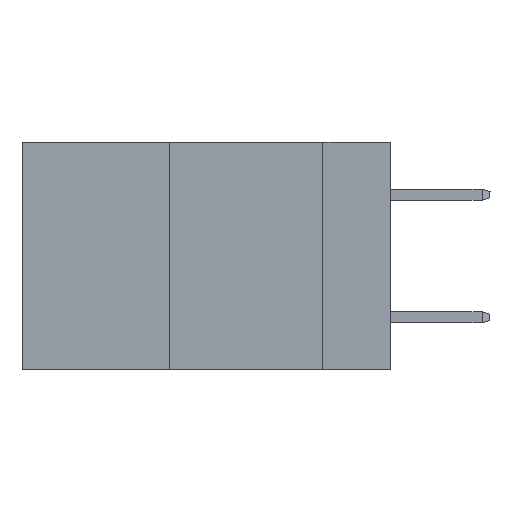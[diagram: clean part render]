
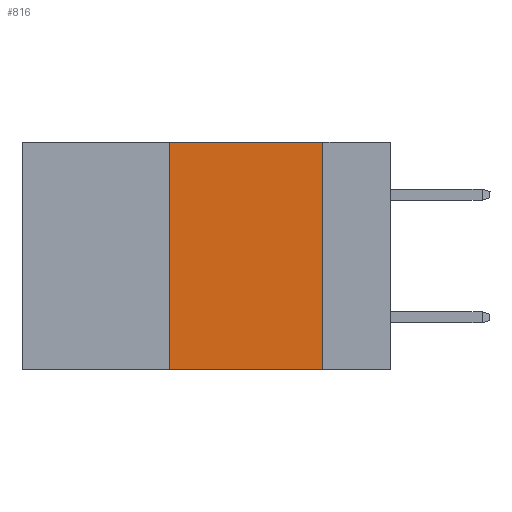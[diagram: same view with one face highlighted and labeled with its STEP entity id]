
A CAD part, left-side view. The second image highlights one B-rep face of the part: STEP entity #816.
In plain terms, the highlighted planar face has unit normal (-1, 0, 0).
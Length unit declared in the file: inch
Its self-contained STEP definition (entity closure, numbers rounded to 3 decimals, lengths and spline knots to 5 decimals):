
#351 = PLANE ( 'NONE',  #15941 ) ;
#454 = EDGE_CURVE ( 'NONE', #11576, #11457, #7574, .T. ) ;
#580 = LINE ( 'NONE', #647, #2822 ) ;
#647 = CARTESIAN_POINT ( 'NONE',  ( 0., 0.6, 0. ) ) ;
#816 = ADVANCED_FACE ( 'NONE', ( #1146 ), #351, .F. ) ;
#1049 = EDGE_LOOP ( 'NONE', ( #15993, #3997, #12586, #17200 ) ) ;
#1146 = FACE_OUTER_BOUND ( 'NONE', #1049, .T. ) ;
#2125 = CARTESIAN_POINT ( 'NONE',  ( 0., 0.36, 0. ) ) ;
#2822 = VECTOR ( 'NONE', #17034, 39.37008 ) ;
#3997 = ORIENTED_EDGE ( 'NONE', *, *, #23733, .F. ) ;
#4300 = LINE ( 'NONE', #9941, #14201 ) ;
#5107 = DIRECTION ( 'NONE',  ( 0., 0., -1. ) ) ;
#5142 = VERTEX_POINT ( 'NONE', #22037 ) ;
#5226 = CARTESIAN_POINT ( 'NONE',  ( 0., 0.36, 0. ) ) ;
#6921 = CARTESIAN_POINT ( 'NONE',  ( 0., 0.36, -0.37 ) ) ;
#7119 = CARTESIAN_POINT ( 'NONE',  ( 0., 0.6, 0. ) ) ;
#7574 = LINE ( 'NONE', #5226, #11432 ) ;
#8896 = DIRECTION ( 'NONE',  ( 0., 0., 1. ) ) ;
#9941 = CARTESIAN_POINT ( 'NONE',  ( 0., 0.6, -0.37 ) ) ;
#10901 = DIRECTION ( 'NONE',  ( 0., 0., -1. ) ) ;
#11087 = EDGE_CURVE ( 'NONE', #19222, #5142, #18822, .T. ) ;
#11153 = DIRECTION ( 'NONE',  ( 1., 0., 0. ) ) ;
#11432 = VECTOR ( 'NONE', #8896, 39.37008 ) ;
#11457 = VERTEX_POINT ( 'NONE', #2125 ) ;
#11576 = VERTEX_POINT ( 'NONE', #6921 ) ;
#12586 = ORIENTED_EDGE ( 'NONE', *, *, #454, .F. ) ;
#14201 = VECTOR ( 'NONE', #18276, 39.37008 ) ;
#15941 = AXIS2_PLACEMENT_3D ( 'NONE', #7119, #11153, #10901 ) ;
#15993 = ORIENTED_EDGE ( 'NONE', *, *, #11087, .F. ) ;
#17034 = DIRECTION ( 'NONE',  ( 0., -1., 0. ) ) ;
#17200 = ORIENTED_EDGE ( 'NONE', *, *, #20209, .T. ) ;
#17271 = CARTESIAN_POINT ( 'NONE',  ( 0., 0.11, 0. ) ) ;
#18276 = DIRECTION ( 'NONE',  ( 0., -1., 0. ) ) ;
#18822 = LINE ( 'NONE', #17271, #21375 ) ;
#19222 = VERTEX_POINT ( 'NONE', #22771 ) ;
#20209 = EDGE_CURVE ( 'NONE', #11576, #5142, #4300, .T. ) ;
#21375 = VECTOR ( 'NONE', #5107, 39.37008 ) ;
#22037 = CARTESIAN_POINT ( 'NONE',  ( 0., 0.11, -0.37 ) ) ;
#22771 = CARTESIAN_POINT ( 'NONE',  ( 0., 0.11, 0. ) ) ;
#23733 = EDGE_CURVE ( 'NONE', #11457, #19222, #580, .T. ) ;
